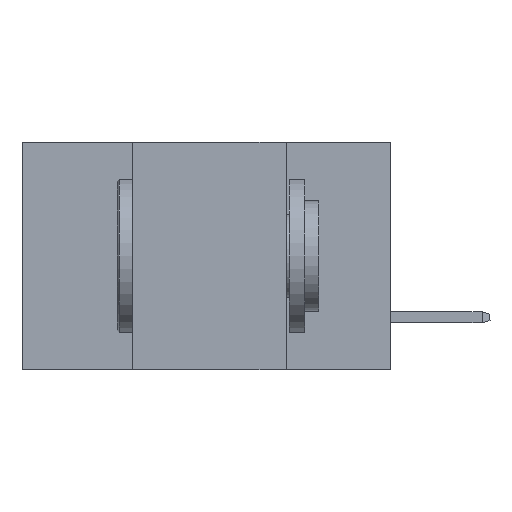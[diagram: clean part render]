
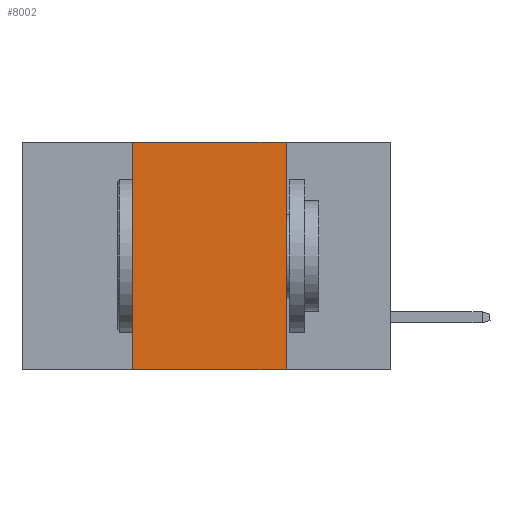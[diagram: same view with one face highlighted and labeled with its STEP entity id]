
A CAD part, left-side view. The second image highlights one B-rep face of the part: STEP entity #8002.
In plain terms, the highlighted planar face has unit normal (-1, 0, 0).
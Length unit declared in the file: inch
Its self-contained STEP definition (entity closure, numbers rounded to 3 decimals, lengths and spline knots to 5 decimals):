
#62 = CARTESIAN_POINT ( 'NONE',  ( 0., 0.42, -0.37 ) ) ;
#478 = AXIS2_PLACEMENT_3D ( 'NONE', #1644, #5370, #3079 ) ;
#1218 = LINE ( 'NONE', #1257, #1934 ) ;
#1257 = CARTESIAN_POINT ( 'NONE',  ( 0., 0.17, 0. ) ) ;
#1417 = CARTESIAN_POINT ( 'NONE',  ( 0., 0.42, 0. ) ) ;
#1644 = CARTESIAN_POINT ( 'NONE',  ( 0., 0.6, 0. ) ) ;
#1775 = VERTEX_POINT ( 'NONE', #62 ) ;
#1934 = VECTOR ( 'NONE', #3494, 39.37008 ) ;
#2462 = VERTEX_POINT ( 'NONE', #1417 ) ;
#2606 = EDGE_CURVE ( 'NONE', #1775, #2462, #6660, .T. ) ;
#2980 = CARTESIAN_POINT ( 'NONE',  ( 0., 0.42, 0. ) ) ;
#3015 = ORIENTED_EDGE ( 'NONE', *, *, #5421, .F. ) ;
#3040 = PLANE ( 'NONE',  #478 ) ;
#3079 = DIRECTION ( 'NONE',  ( 0., 0., -1. ) ) ;
#3344 = CARTESIAN_POINT ( 'NONE',  ( 0., 0.17, -0.37 ) ) ;
#3489 = ORIENTED_EDGE ( 'NONE', *, *, #5480, .T. ) ;
#3494 = DIRECTION ( 'NONE',  ( 0., 0., -1. ) ) ;
#3614 = VECTOR ( 'NONE', #5339, 39.37008 ) ;
#3802 = CARTESIAN_POINT ( 'NONE',  ( 0., 0.6, 0. ) ) ;
#4154 = DIRECTION ( 'NONE',  ( 0., -1., 0. ) ) ;
#4702 = ORIENTED_EDGE ( 'NONE', *, *, #2606, .F. ) ;
#4878 = CARTESIAN_POINT ( 'NONE',  ( 0., 0.6, -0.37 ) ) ;
#5329 = VECTOR ( 'NONE', #6751, 39.37008 ) ;
#5339 = DIRECTION ( 'NONE',  ( 0., -1., 0. ) ) ;
#5368 = VERTEX_POINT ( 'NONE', #3344 ) ;
#5370 = DIRECTION ( 'NONE',  ( 1., 0., 0. ) ) ;
#5421 = EDGE_CURVE ( 'NONE', #9491, #5368, #1218, .T. ) ;
#5480 = EDGE_CURVE ( 'NONE', #1775, #5368, #5642, .T. ) ;
#5642 = LINE ( 'NONE', #4878, #8331 ) ;
#6660 = LINE ( 'NONE', #2980, #5329 ) ;
#6751 = DIRECTION ( 'NONE',  ( 0., 0., 1. ) ) ;
#7665 = EDGE_LOOP ( 'NONE', ( #3015, #8063, #4702, #3489 ) ) ;
#7840 = LINE ( 'NONE', #3802, #3614 ) ;
#7964 = EDGE_CURVE ( 'NONE', #2462, #9491, #7840, .T. ) ;
#8002 = ADVANCED_FACE ( 'NONE', ( #8171 ), #3040, .F. ) ;
#8063 = ORIENTED_EDGE ( 'NONE', *, *, #7964, .F. ) ;
#8171 = FACE_OUTER_BOUND ( 'NONE', #7665, .T. ) ;
#8331 = VECTOR ( 'NONE', #4154, 39.37008 ) ;
#8681 = CARTESIAN_POINT ( 'NONE',  ( 0., 0.17, 0. ) ) ;
#9491 = VERTEX_POINT ( 'NONE', #8681 ) ;
